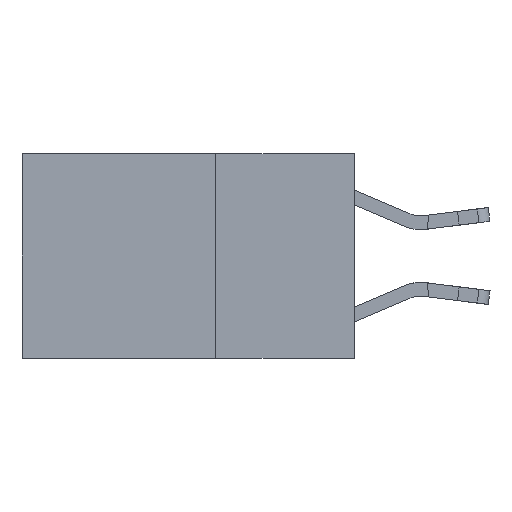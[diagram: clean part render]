
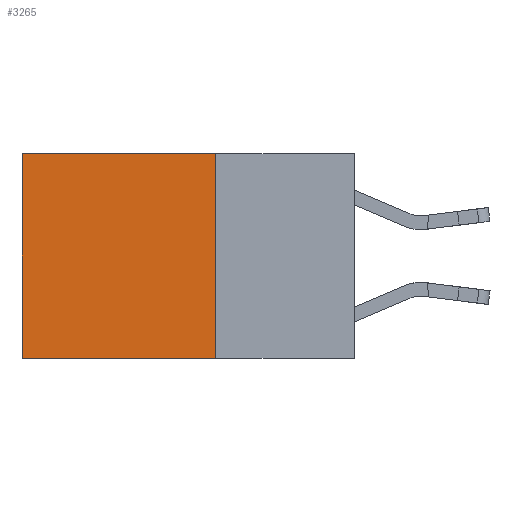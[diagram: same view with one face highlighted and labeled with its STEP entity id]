
A CAD part, left-side view. The second image highlights one B-rep face of the part: STEP entity #3265.
In plain terms, the highlighted planar face has unit normal (-1, 0, 0).
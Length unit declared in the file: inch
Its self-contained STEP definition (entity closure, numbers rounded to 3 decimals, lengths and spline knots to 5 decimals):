
#519 = CARTESIAN_POINT ( 'NONE',  ( 0.2625, 0.25, -0.37 ) ) ;
#1122 = FACE_OUTER_BOUND ( 'NONE', #13099, .T. ) ;
#1427 = CARTESIAN_POINT ( 'NONE',  ( 0.2625, 0.6, 0. ) ) ;
#1829 = CARTESIAN_POINT ( 'NONE',  ( 0.2625, 0.25, 0. ) ) ;
#2041 = EDGE_CURVE ( 'NONE', #5480, #7090, #7140, .T. ) ;
#2951 = DIRECTION ( 'NONE',  ( 0., 1., 0. ) ) ;
#3265 = ADVANCED_FACE ( 'NONE', ( #1122 ), #14328, .F. ) ;
#5203 = EDGE_CURVE ( 'NONE', #14432, #12279, #13041, .T. ) ;
#5480 = VERTEX_POINT ( 'NONE', #16222 ) ;
#5627 = DIRECTION ( 'NONE',  ( 0., 0., -1. ) ) ;
#5888 = VECTOR ( 'NONE', #2951, 39.37008 ) ;
#6692 = ORIENTED_EDGE ( 'NONE', *, *, #5203, .T. ) ;
#7090 = VERTEX_POINT ( 'NONE', #519 ) ;
#7140 = LINE ( 'NONE', #8993, #16519 ) ;
#7266 = DIRECTION ( 'NONE',  ( 0., 1., 0. ) ) ;
#7788 = EDGE_CURVE ( 'NONE', #5480, #14432, #11760, .T. ) ;
#7897 = ORIENTED_EDGE ( 'NONE', *, *, #7788, .T. ) ;
#7947 = DIRECTION ( 'NONE',  ( 0., 0., -1. ) ) ;
#8993 = CARTESIAN_POINT ( 'NONE',  ( 0.2625, 0.25, 0. ) ) ;
#9566 = CARTESIAN_POINT ( 'NONE',  ( 0.2625, 0.6, -0.37 ) ) ;
#10269 = DIRECTION ( 'NONE',  ( 0., 0., -1. ) ) ;
#10384 = CARTESIAN_POINT ( 'NONE',  ( 0.2625, 0.25, 0. ) ) ;
#10536 = AXIS2_PLACEMENT_3D ( 'NONE', #10384, #15588, #7947 ) ;
#10786 = CARTESIAN_POINT ( 'NONE',  ( 0.2625, 0.25, -0.37 ) ) ;
#10884 = ORIENTED_EDGE ( 'NONE', *, *, #2041, .F. ) ;
#11760 = LINE ( 'NONE', #1829, #12168 ) ;
#12168 = VECTOR ( 'NONE', #7266, 39.37008 ) ;
#12279 = VERTEX_POINT ( 'NONE', #9566 ) ;
#13041 = LINE ( 'NONE', #1427, #15617 ) ;
#13099 = EDGE_LOOP ( 'NONE', ( #6692, #13905, #10884, #7897 ) ) ;
#13905 = ORIENTED_EDGE ( 'NONE', *, *, #14697, .F. ) ;
#14227 = CARTESIAN_POINT ( 'NONE',  ( 0.2625, 0.6, 0. ) ) ;
#14328 = PLANE ( 'NONE',  #10536 ) ;
#14432 = VERTEX_POINT ( 'NONE', #14227 ) ;
#14697 = EDGE_CURVE ( 'NONE', #7090, #12279, #16066, .T. ) ;
#15588 = DIRECTION ( 'NONE',  ( 1., 0., 0. ) ) ;
#15617 = VECTOR ( 'NONE', #5627, 39.37008 ) ;
#16066 = LINE ( 'NONE', #10786, #5888 ) ;
#16222 = CARTESIAN_POINT ( 'NONE',  ( 0.2625, 0.25, 0. ) ) ;
#16519 = VECTOR ( 'NONE', #10269, 39.37008 ) ;
